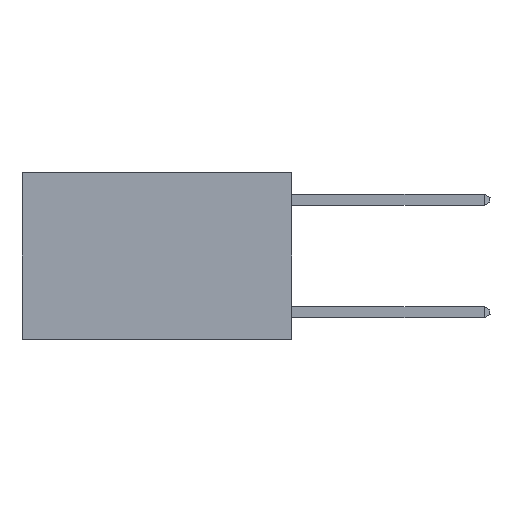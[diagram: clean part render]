
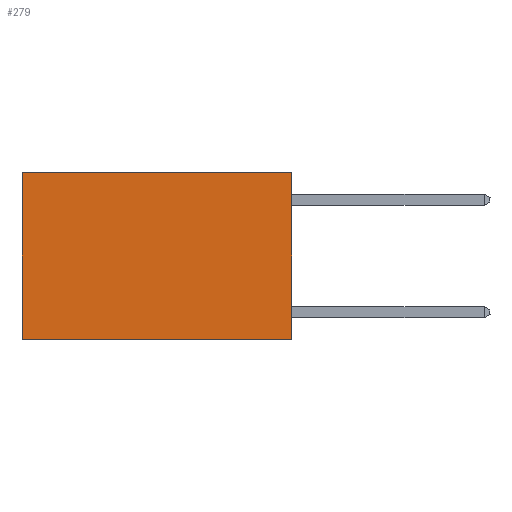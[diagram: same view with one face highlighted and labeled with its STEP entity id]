
A CAD part, left-side view. The second image highlights one B-rep face of the part: STEP entity #279.
In plain terms, the highlighted planar face has unit normal (-1, 0, 0).
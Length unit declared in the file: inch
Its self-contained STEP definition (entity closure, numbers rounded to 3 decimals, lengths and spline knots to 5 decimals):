
#279 = ADVANCED_FACE ( 'NONE', ( #1511 ), #10852, .F. ) ;
#333 = VECTOR ( 'NONE', #10929, 39.37008 ) ;
#382 = CARTESIAN_POINT ( 'NONE',  ( 0.2625, 0.6, -0.37 ) ) ;
#383 = CARTESIAN_POINT ( 'NONE',  ( 0.2625, 0., 0. ) ) ;
#861 = ORIENTED_EDGE ( 'NONE', *, *, #7379, .F. ) ;
#934 = DIRECTION ( 'NONE',  ( 0., 1., 0. ) ) ;
#1416 = ORIENTED_EDGE ( 'NONE', *, *, #1776, .T. ) ;
#1511 = FACE_OUTER_BOUND ( 'NONE', #11850, .T. ) ;
#1776 = EDGE_CURVE ( 'NONE', #10295, #7555, #12060, .T. ) ;
#1804 = EDGE_CURVE ( 'NONE', #2758, #5812, #13061, .T. ) ;
#1906 = CARTESIAN_POINT ( 'NONE',  ( 0.2625, 0., 0. ) ) ;
#2758 = VERTEX_POINT ( 'NONE', #7099 ) ;
#2887 = VECTOR ( 'NONE', #7997, 39.37008 ) ;
#4102 = EDGE_CURVE ( 'NONE', #2758, #10295, #10078, .T. ) ;
#4276 = AXIS2_PLACEMENT_3D ( 'NONE', #383, #4712, #8536 ) ;
#4712 = DIRECTION ( 'NONE',  ( 1., 0., 0. ) ) ;
#4923 = CARTESIAN_POINT ( 'NONE',  ( 0.2625, 0.6, 0. ) ) ;
#5812 = VERTEX_POINT ( 'NONE', #8132 ) ;
#6401 = VECTOR ( 'NONE', #8968, 39.37008 ) ;
#7099 = CARTESIAN_POINT ( 'NONE',  ( 0.2625, 0., 0. ) ) ;
#7379 = EDGE_CURVE ( 'NONE', #5812, #7555, #12770, .T. ) ;
#7555 = VERTEX_POINT ( 'NONE', #382 ) ;
#7997 = DIRECTION ( 'NONE',  ( 0., 0., -1. ) ) ;
#8132 = CARTESIAN_POINT ( 'NONE',  ( 0.2625, 0., -0.37 ) ) ;
#8536 = DIRECTION ( 'NONE',  ( 0., 0., -1. ) ) ;
#8968 = DIRECTION ( 'NONE',  ( 0., 1., 0. ) ) ;
#10078 = LINE ( 'NONE', #12204, #12995 ) ;
#10295 = VERTEX_POINT ( 'NONE', #13016 ) ;
#10852 = PLANE ( 'NONE',  #4276 ) ;
#10929 = DIRECTION ( 'NONE',  ( 0., 0., -1. ) ) ;
#11537 = ORIENTED_EDGE ( 'NONE', *, *, #1804, .F. ) ;
#11850 = EDGE_LOOP ( 'NONE', ( #1416, #861, #11537, #12931 ) ) ;
#11973 = CARTESIAN_POINT ( 'NONE',  ( 0.2625, 0., -0.37 ) ) ;
#12060 = LINE ( 'NONE', #4923, #2887 ) ;
#12204 = CARTESIAN_POINT ( 'NONE',  ( 0.2625, 0., 0. ) ) ;
#12770 = LINE ( 'NONE', #11973, #6401 ) ;
#12931 = ORIENTED_EDGE ( 'NONE', *, *, #4102, .T. ) ;
#12995 = VECTOR ( 'NONE', #934, 39.37008 ) ;
#13016 = CARTESIAN_POINT ( 'NONE',  ( 0.2625, 0.6, 0. ) ) ;
#13061 = LINE ( 'NONE', #1906, #333 ) ;
